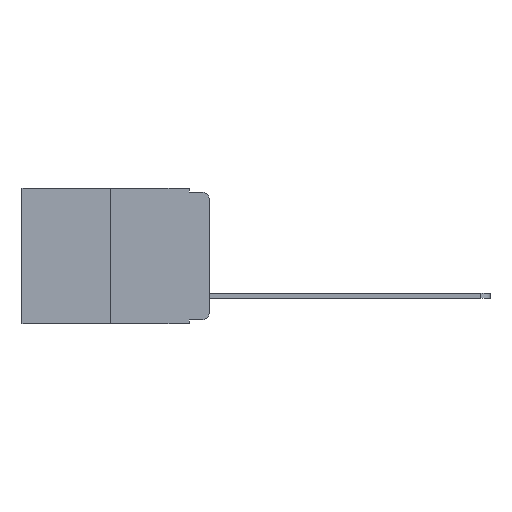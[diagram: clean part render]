
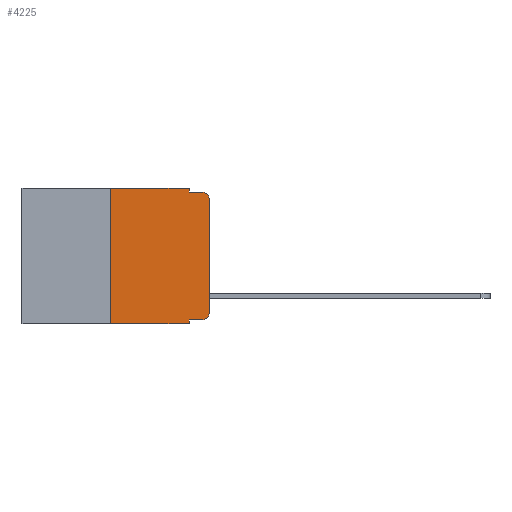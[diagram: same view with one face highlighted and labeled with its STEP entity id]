
A CAD part, left-side view. The second image highlights one B-rep face of the part: STEP entity #4225.
In plain terms, the highlighted planar face has unit normal (-1, 0, 0).
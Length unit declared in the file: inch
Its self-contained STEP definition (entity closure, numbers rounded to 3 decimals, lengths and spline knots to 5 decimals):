
#211 = CARTESIAN_POINT ( 'NONE',  ( 0., 0.051, 0. ) ) ;
#392 = DIRECTION ( 'NONE',  ( 0., -1., 0. ) ) ;
#641 = CARTESIAN_POINT ( 'NONE',  ( 0., 0.25, -0.343 ) ) ;
#726 = VECTOR ( 'NONE', #13587, 39.37008 ) ;
#731 = CARTESIAN_POINT ( 'NONE',  ( 0., 0.02, -0.333 ) ) ;
#857 = VERTEX_POINT ( 'NONE', #13137 ) ;
#1084 = VECTOR ( 'NONE', #14444, 39.37008 ) ;
#1735 = DIRECTION ( 'NONE',  ( 0., 0., 1. ) ) ;
#1814 = ORIENTED_EDGE ( 'NONE', *, *, #1816, .F. ) ;
#1816 = EDGE_CURVE ( 'NONE', #8049, #857, #13626, .T. ) ;
#1897 = VERTEX_POINT ( 'NONE', #13351 ) ;
#2206 = ORIENTED_EDGE ( 'NONE', *, *, #4441, .F. ) ;
#2410 = EDGE_CURVE ( 'NONE', #7527, #10904, #10189, .T. ) ;
#3115 = LINE ( 'NONE', #4201, #8863 ) ;
#3632 = CARTESIAN_POINT ( 'NONE',  ( 0., 0.473, -0.343 ) ) ;
#3824 = VECTOR ( 'NONE', #5731, 39.37008 ) ;
#4059 = LINE ( 'NONE', #211, #6758 ) ;
#4150 = DIRECTION ( 'NONE',  ( 0., 0., -1. ) ) ;
#4201 = CARTESIAN_POINT ( 'NONE',  ( 0., 0.473, 0. ) ) ;
#4225 = ADVANCED_FACE ( 'NONE', ( #9244 ), #13388, .F. ) ;
#4335 = LINE ( 'NONE', #4860, #726 ) ;
#4429 = VECTOR ( 'NONE', #1735, 39.37008 ) ;
#4441 = EDGE_CURVE ( 'NONE', #12755, #8049, #4059, .T. ) ;
#4577 = EDGE_CURVE ( 'NONE', #12605, #10904, #13350, .T. ) ;
#4714 = EDGE_CURVE ( 'NONE', #13338, #12755, #3115, .T. ) ;
#4815 = EDGE_CURVE ( 'NONE', #12605, #13338, #7441, .T. ) ;
#4860 = CARTESIAN_POINT ( 'NONE',  ( 0., 0.051, -0.333 ) ) ;
#4936 = VECTOR ( 'NONE', #9078, 39.37008 ) ;
#5001 = DIRECTION ( 'NONE',  ( -1., 0., 0. ) ) ;
#5051 = AXIS2_PLACEMENT_3D ( 'NONE', #13412, #6954, #6933 ) ;
#5082 = AXIS2_PLACEMENT_3D ( 'NONE', #5615, #5001, #11908 ) ;
#5615 = CARTESIAN_POINT ( 'NONE',  ( 0., 0.02, -0.03 ) ) ;
#5731 = DIRECTION ( 'NONE',  ( 0., 0., -1. ) ) ;
#5806 = CARTESIAN_POINT ( 'NONE',  ( 0., 0.051, 0. ) ) ;
#6317 = CARTESIAN_POINT ( 'NONE',  ( 0., 0.02, -0.313 ) ) ;
#6468 = CARTESIAN_POINT ( 'NONE',  ( 0., 0.25, 0. ) ) ;
#6559 = EDGE_CURVE ( 'NONE', #1897, #857, #8804, .T. ) ;
#6758 = VECTOR ( 'NONE', #4150, 39.37008 ) ;
#6933 = DIRECTION ( 'NONE',  ( 0., 0., -1. ) ) ;
#6954 = DIRECTION ( 'NONE',  ( 1., 0., 0. ) ) ;
#7333 = LINE ( 'NONE', #13410, #1084 ) ;
#7437 = DIRECTION ( 'NONE',  ( 0., 0., -1. ) ) ;
#7441 = LINE ( 'NONE', #6468, #4429 ) ;
#7527 = VERTEX_POINT ( 'NONE', #8033 ) ;
#7566 = EDGE_LOOP ( 'NONE', ( #10261, #7652, #1814, #2206, #14016, #8722, #9086, #9439, #12591, #10426 ) ) ;
#7652 = ORIENTED_EDGE ( 'NONE', *, *, #6559, .T. ) ;
#8033 = CARTESIAN_POINT ( 'NONE',  ( 0., 0.051, -0.333 ) ) ;
#8049 = VERTEX_POINT ( 'NONE', #12122 ) ;
#8722 = ORIENTED_EDGE ( 'NONE', *, *, #4815, .F. ) ;
#8804 = CIRCLE ( 'NONE', #5082, 0.02 ) ;
#8816 = EDGE_CURVE ( 'NONE', #12965, #1897, #7333, .T. ) ;
#8863 = VECTOR ( 'NONE', #392, 39.37008 ) ;
#9078 = DIRECTION ( 'NONE',  ( 0., -1., 0. ) ) ;
#9086 = ORIENTED_EDGE ( 'NONE', *, *, #4577, .T. ) ;
#9244 = FACE_OUTER_BOUND ( 'NONE', #7566, .T. ) ;
#9439 = ORIENTED_EDGE ( 'NONE', *, *, #2410, .F. ) ;
#10189 = LINE ( 'NONE', #5806, #3824 ) ;
#10261 = ORIENTED_EDGE ( 'NONE', *, *, #8816, .T. ) ;
#10401 = CARTESIAN_POINT ( 'NONE',  ( 0., 0.25, 0. ) ) ;
#10426 = ORIENTED_EDGE ( 'NONE', *, *, #12483, .T. ) ;
#10555 = VECTOR ( 'NONE', #11011, 39.37008 ) ;
#10601 = CARTESIAN_POINT ( 'NONE',  ( 0., 0.051, -0.01 ) ) ;
#10904 = VERTEX_POINT ( 'NONE', #11137 ) ;
#11011 = DIRECTION ( 'NONE',  ( 0., -1., 0. ) ) ;
#11137 = CARTESIAN_POINT ( 'NONE',  ( 0., 0.051, -0.343 ) ) ;
#11459 = VERTEX_POINT ( 'NONE', #731 ) ;
#11632 = AXIS2_PLACEMENT_3D ( 'NONE', #6317, #13860, #7437 ) ;
#11908 = DIRECTION ( 'NONE',  ( 0., 0., -1. ) ) ;
#12122 = CARTESIAN_POINT ( 'NONE',  ( 0., 0.051, -0.01 ) ) ;
#12483 = EDGE_CURVE ( 'NONE', #11459, #12965, #12489, .T. ) ;
#12489 = CIRCLE ( 'NONE', #11632, 0.02 ) ;
#12591 = ORIENTED_EDGE ( 'NONE', *, *, #13839, .T. ) ;
#12605 = VERTEX_POINT ( 'NONE', #641 ) ;
#12755 = VERTEX_POINT ( 'NONE', #14342 ) ;
#12965 = VERTEX_POINT ( 'NONE', #13958 ) ;
#13137 = CARTESIAN_POINT ( 'NONE',  ( 0., 0.02, -0.01 ) ) ;
#13338 = VERTEX_POINT ( 'NONE', #10401 ) ;
#13350 = LINE ( 'NONE', #3632, #10555 ) ;
#13351 = CARTESIAN_POINT ( 'NONE',  ( 0., 0., -0.03 ) ) ;
#13388 = PLANE ( 'NONE',  #5051 ) ;
#13410 = CARTESIAN_POINT ( 'NONE',  ( 0., 0., 0. ) ) ;
#13412 = CARTESIAN_POINT ( 'NONE',  ( 0., 0.473, 0. ) ) ;
#13587 = DIRECTION ( 'NONE',  ( 0., -1., 0. ) ) ;
#13626 = LINE ( 'NONE', #10601, #4936 ) ;
#13839 = EDGE_CURVE ( 'NONE', #7527, #11459, #4335, .T. ) ;
#13860 = DIRECTION ( 'NONE',  ( -1., 0., 0. ) ) ;
#13958 = CARTESIAN_POINT ( 'NONE',  ( 0., 0., -0.313 ) ) ;
#14016 = ORIENTED_EDGE ( 'NONE', *, *, #4714, .F. ) ;
#14342 = CARTESIAN_POINT ( 'NONE',  ( 0., 0.051, 0. ) ) ;
#14444 = DIRECTION ( 'NONE',  ( 0., 0., 1. ) ) ;
